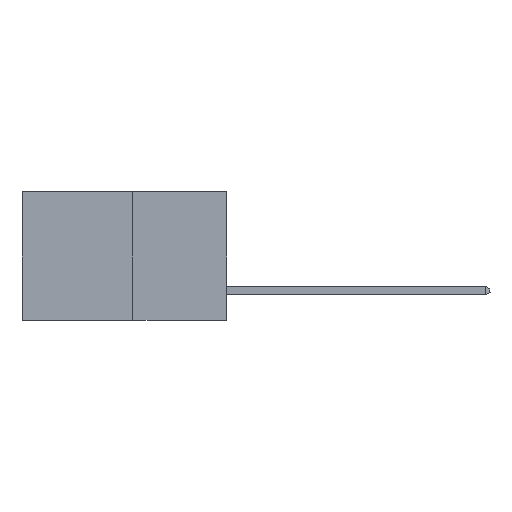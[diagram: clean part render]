
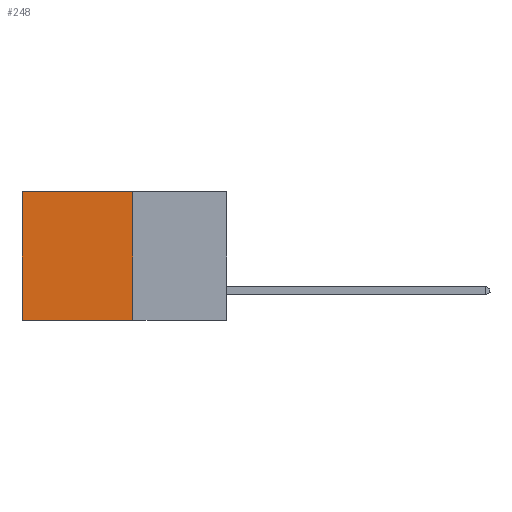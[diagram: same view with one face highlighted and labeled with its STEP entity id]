
A CAD part, left-side view. The second image highlights one B-rep face of the part: STEP entity #248.
In plain terms, the highlighted planar face has unit normal (-1, 0, 0).
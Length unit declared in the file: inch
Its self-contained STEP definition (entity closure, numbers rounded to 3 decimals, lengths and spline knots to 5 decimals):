
#248 = ADVANCED_FACE ( 'NONE', ( #17366 ), #19007, .F. ) ;
#416 = EDGE_CURVE ( 'NONE', #17055, #17214, #18210, .T. ) ;
#439 = VERTEX_POINT ( 'NONE', #9760 ) ;
#901 = LINE ( 'NONE', #22535, #1441 ) ;
#1441 = VECTOR ( 'NONE', #6224, 39.37008 ) ;
#1794 = AXIS2_PLACEMENT_3D ( 'NONE', #19319, #17977, #4353 ) ;
#3673 = VECTOR ( 'NONE', #18939, 39.37008 ) ;
#4353 = DIRECTION ( 'NONE',  ( 0., 0., -1. ) ) ;
#4822 = VERTEX_POINT ( 'NONE', #22519 ) ;
#5369 = EDGE_LOOP ( 'NONE', ( #6477, #11455, #17192, #13791 ) ) ;
#6224 = DIRECTION ( 'NONE',  ( 0., 1., 0. ) ) ;
#6251 = DIRECTION ( 'NONE',  ( 0., 0., -1. ) ) ;
#6477 = ORIENTED_EDGE ( 'NONE', *, *, #416, .T. ) ;
#7313 = LINE ( 'NONE', #17030, #16387 ) ;
#7733 = EDGE_CURVE ( 'NONE', #439, #4822, #7313, .T. ) ;
#8473 = DIRECTION ( 'NONE',  ( 0., 0., -1. ) ) ;
#8575 = CARTESIAN_POINT ( 'NONE',  ( 0.277, 0.59, -0.37 ) ) ;
#9116 = CARTESIAN_POINT ( 'NONE',  ( 0.277, 0.59, 0. ) ) ;
#9760 = CARTESIAN_POINT ( 'NONE',  ( 0.277, 0.27, 0. ) ) ;
#11455 = ORIENTED_EDGE ( 'NONE', *, *, #21233, .F. ) ;
#13521 = CARTESIAN_POINT ( 'NONE',  ( 0.277, 0.27, -0.37 ) ) ;
#13791 = ORIENTED_EDGE ( 'NONE', *, *, #17375, .T. ) ;
#16387 = VECTOR ( 'NONE', #6251, 39.37008 ) ;
#17030 = CARTESIAN_POINT ( 'NONE',  ( 0.277, 0.27, -0.37 ) ) ;
#17055 = VERTEX_POINT ( 'NONE', #9116 ) ;
#17192 = ORIENTED_EDGE ( 'NONE', *, *, #7733, .F. ) ;
#17214 = VERTEX_POINT ( 'NONE', #22149 ) ;
#17366 = FACE_OUTER_BOUND ( 'NONE', #5369, .T. ) ;
#17375 = EDGE_CURVE ( 'NONE', #439, #17055, #901, .T. ) ;
#17977 = DIRECTION ( 'NONE',  ( 1., 0., 0. ) ) ;
#18185 = LINE ( 'NONE', #13521, #3673 ) ;
#18210 = LINE ( 'NONE', #8575, #21814 ) ;
#18939 = DIRECTION ( 'NONE',  ( 0., 1., 0. ) ) ;
#19007 = PLANE ( 'NONE',  #1794 ) ;
#19319 = CARTESIAN_POINT ( 'NONE',  ( 0.277, 0.27, -0.37 ) ) ;
#21233 = EDGE_CURVE ( 'NONE', #4822, #17214, #18185, .T. ) ;
#21814 = VECTOR ( 'NONE', #8473, 39.37008 ) ;
#22149 = CARTESIAN_POINT ( 'NONE',  ( 0.277, 0.59, -0.37 ) ) ;
#22519 = CARTESIAN_POINT ( 'NONE',  ( 0.277, 0.27, -0.37 ) ) ;
#22535 = CARTESIAN_POINT ( 'NONE',  ( 0.277, 0.27, 0. ) ) ;
